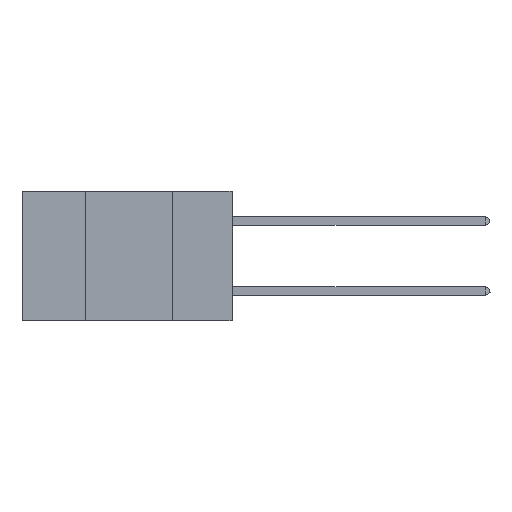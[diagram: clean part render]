
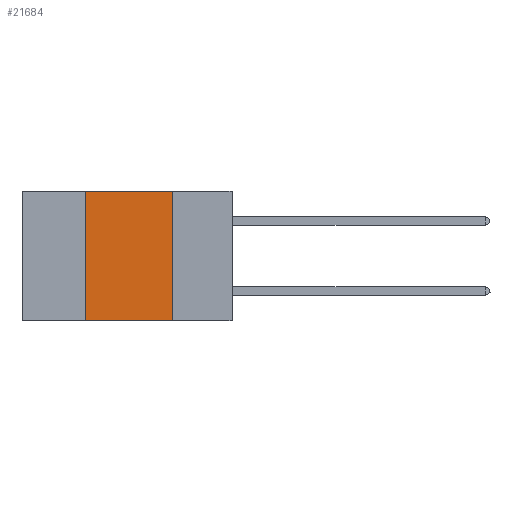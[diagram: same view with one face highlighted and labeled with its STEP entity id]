
A CAD part, left-side view. The second image highlights one B-rep face of the part: STEP entity #21684.
In plain terms, the highlighted planar face has unit normal (-1, 0, 0).
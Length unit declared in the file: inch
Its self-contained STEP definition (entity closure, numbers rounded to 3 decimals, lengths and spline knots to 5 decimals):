
#167 = EDGE_CURVE ( 'NONE', #21567, #30284, #1127, .T. ) ;
#705 = DIRECTION ( 'NONE',  ( 0., 0., 1. ) ) ;
#1127 = LINE ( 'NONE', #33049, #16920 ) ;
#2635 = EDGE_CURVE ( 'NONE', #30284, #18903, #28218, .T. ) ;
#2829 = LINE ( 'NONE', #27182, #5335 ) ;
#2840 = ORIENTED_EDGE ( 'NONE', *, *, #19616, .F. ) ;
#4421 = VECTOR ( 'NONE', #7546, 39.37008 ) ;
#4655 = CARTESIAN_POINT ( 'NONE',  ( 0., 0.42, -0.37 ) ) ;
#5335 = VECTOR ( 'NONE', #705, 39.37008 ) ;
#5433 = AXIS2_PLACEMENT_3D ( 'NONE', #5629, #32272, #13340 ) ;
#5629 = CARTESIAN_POINT ( 'NONE',  ( 0., 0.6, 0. ) ) ;
#7278 = DIRECTION ( 'NONE',  ( 0., -1., 0. ) ) ;
#7546 = DIRECTION ( 'NONE',  ( 0., 0., -1. ) ) ;
#7575 = CARTESIAN_POINT ( 'NONE',  ( 0., 0.42, 0. ) ) ;
#8089 = FACE_OUTER_BOUND ( 'NONE', #26253, .T. ) ;
#13340 = DIRECTION ( 'NONE',  ( 0., 0., -1. ) ) ;
#16920 = VECTOR ( 'NONE', #17439, 39.37008 ) ;
#17439 = DIRECTION ( 'NONE',  ( 0., -1., 0. ) ) ;
#18069 = CARTESIAN_POINT ( 'NONE',  ( 0., 0.17, 0. ) ) ;
#18903 = VERTEX_POINT ( 'NONE', #28650 ) ;
#19616 = EDGE_CURVE ( 'NONE', #26221, #21567, #2829, .T. ) ;
#21567 = VERTEX_POINT ( 'NONE', #7575 ) ;
#21684 = ADVANCED_FACE ( 'NONE', ( #8089 ), #32440, .F. ) ;
#22077 = ORIENTED_EDGE ( 'NONE', *, *, #24238, .T. ) ;
#22876 = LINE ( 'NONE', #31280, #27260 ) ;
#24238 = EDGE_CURVE ( 'NONE', #26221, #18903, #22876, .T. ) ;
#26221 = VERTEX_POINT ( 'NONE', #4655 ) ;
#26253 = EDGE_LOOP ( 'NONE', ( #33967, #26568, #2840, #22077 ) ) ;
#26568 = ORIENTED_EDGE ( 'NONE', *, *, #167, .F. ) ;
#27182 = CARTESIAN_POINT ( 'NONE',  ( 0., 0.42, 0. ) ) ;
#27260 = VECTOR ( 'NONE', #7278, 39.37008 ) ;
#28218 = LINE ( 'NONE', #18069, #4421 ) ;
#28650 = CARTESIAN_POINT ( 'NONE',  ( 0., 0.17, -0.37 ) ) ;
#30284 = VERTEX_POINT ( 'NONE', #34030 ) ;
#31280 = CARTESIAN_POINT ( 'NONE',  ( 0., 0.6, -0.37 ) ) ;
#32272 = DIRECTION ( 'NONE',  ( 1., 0., 0. ) ) ;
#32440 = PLANE ( 'NONE',  #5433 ) ;
#33049 = CARTESIAN_POINT ( 'NONE',  ( 0., 0.6, 0. ) ) ;
#33967 = ORIENTED_EDGE ( 'NONE', *, *, #2635, .F. ) ;
#34030 = CARTESIAN_POINT ( 'NONE',  ( 0., 0.17, 0. ) ) ;
